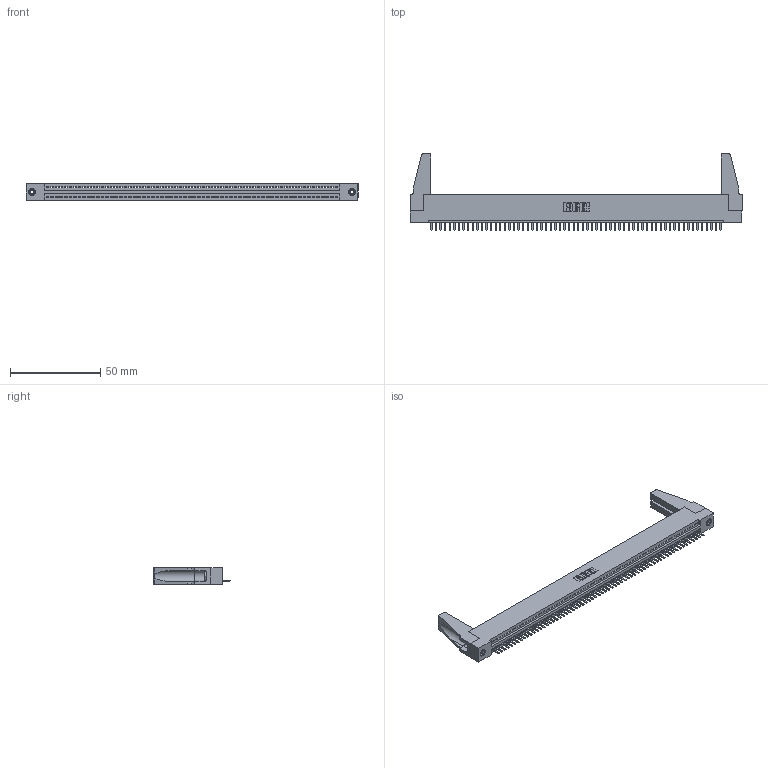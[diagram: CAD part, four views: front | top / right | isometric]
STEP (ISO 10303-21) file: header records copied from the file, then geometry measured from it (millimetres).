
FILE_DESCRIPTION (( 'STEP AP203' ), '1' );
FILE_NAME ('345-064-520-188.STEP', '2019-10-11T13:35:16', ( '' ), ( '' ), 'SwSTEP 2.0', 'SolidWorks 2016', '' );
FILE_SCHEMA (( 'CONFIG_CONTROL_DESIGN' ));
Length unit declared in the file: inch
Products named in the file (5): 345 Part_Flush Mounting Lugs - 0.156 Dia-TH; 345-220-078_345-220-088; 345-064-520-188; 345-250-001_345-250-001-102; 345-292-001_345-293-120
Assembly tree (69 placements, depth 2):
  345-064-520-188
    345 Part_Flush Mounting Lugs - 0.156 Dia-TH
    345-292-001_345-293-120  x64
    345-250-001_345-250-001-102  x2
    345-220-078_345-220-088  x2
Bounding box: 183.79 x 42.55 x 9.4 mm (x, y, z)
Volume: 20705.6 mm3; surface area: 26019.6 mm2
Topology: 69 solids, 69 shells, 4218 faces, 12431 edges, 8106 vertices
Faces by surface type: plane 2840, cylinder 1362, cone 12, torus 4
Entity records: 47468 total; most frequent: CARTESIAN_POINT 8222, ORIENTED_EDGE 8168, DIRECTION 7144, EDGE_CURVE 4084, VECTOR 3650, LINE 3650, VERTEX_POINT 2714, AXIS2_PLACEMENT_3D 1747
